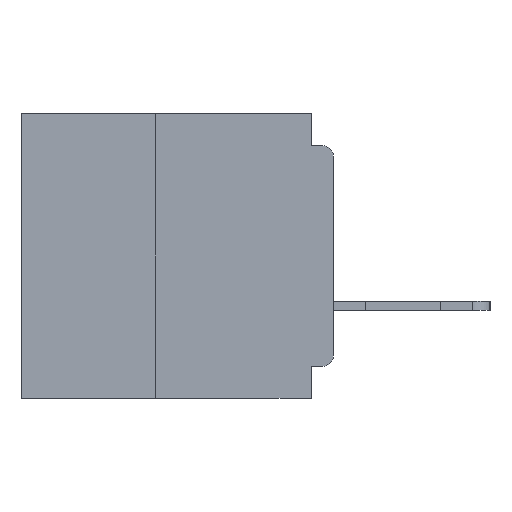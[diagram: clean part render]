
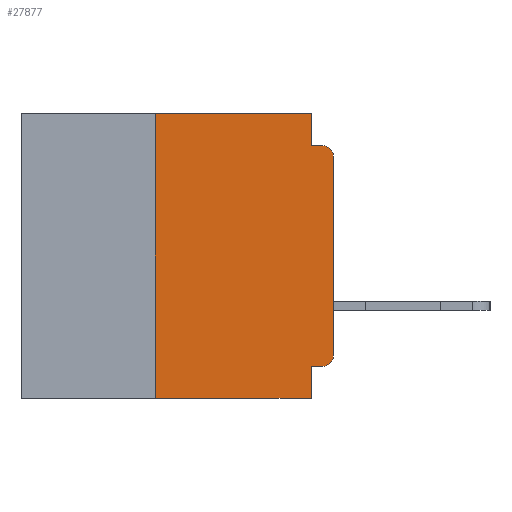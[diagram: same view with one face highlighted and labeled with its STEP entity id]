
A CAD part, left-side view. The second image highlights one B-rep face of the part: STEP entity #27877.
In plain terms, the highlighted planar face has unit normal (-1, 0, 0).
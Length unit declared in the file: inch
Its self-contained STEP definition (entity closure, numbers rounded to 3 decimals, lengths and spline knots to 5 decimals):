
#2453 = DIRECTION ( 'NONE',  ( 0., 0., -1. ) ) ;
#2517 = LINE ( 'NONE', #8392, #47745 ) ;
#2806 = VERTEX_POINT ( 'NONE', #10183 ) ;
#2852 = CARTESIAN_POINT ( 'NONE',  ( 0., 0.25, 0. ) ) ;
#3042 = ORIENTED_EDGE ( 'NONE', *, *, #9630, .F. ) ;
#3552 = DIRECTION ( 'NONE',  ( 0., 0., -1. ) ) ;
#3826 = VERTEX_POINT ( 'NONE', #6297 ) ;
#5851 = LINE ( 'NONE', #14677, #27881 ) ;
#5991 = LINE ( 'NONE', #32245, #39571 ) ;
#6101 = VECTOR ( 'NONE', #44183, 39.37008 ) ;
#6297 = CARTESIAN_POINT ( 'NONE',  ( 0., 0.031, -0.355 ) ) ;
#6954 = VECTOR ( 'NONE', #3552, 39.37008 ) ;
#7157 = DIRECTION ( 'NONE',  ( 1., 0., 0. ) ) ;
#7499 = LINE ( 'NONE', #39809, #6101 ) ;
#8038 = CARTESIAN_POINT ( 'NONE',  ( 0., 0.031, 0. ) ) ;
#8392 = CARTESIAN_POINT ( 'NONE',  ( 0., 0.437, -0.4 ) ) ;
#9630 = EDGE_CURVE ( 'NONE', #53029, #47740, #51088, .T. ) ;
#10183 = CARTESIAN_POINT ( 'NONE',  ( 0., 0., -0.06 ) ) ;
#11050 = LINE ( 'NONE', #43414, #21374 ) ;
#11082 = CARTESIAN_POINT ( 'NONE',  ( 0., 0., -0.34 ) ) ;
#11758 = EDGE_CURVE ( 'NONE', #47740, #37006, #5851, .T. ) ;
#13208 = CARTESIAN_POINT ( 'NONE',  ( 0., 0.015, -0.34 ) ) ;
#14677 = CARTESIAN_POINT ( 'NONE',  ( 0., 0.437, 0. ) ) ;
#16245 = EDGE_LOOP ( 'NONE', ( #28525, #27925, #49879, #46525, #18513, #3042, #54844, #49669, #50476, #22809 ) ) ;
#16630 = VERTEX_POINT ( 'NONE', #11082 ) ;
#17593 = DIRECTION ( 'NONE',  ( 0., 0., -1. ) ) ;
#17692 = VECTOR ( 'NONE', #27886, 39.37008 ) ;
#18513 = ORIENTED_EDGE ( 'NONE', *, *, #11758, .F. ) ;
#20259 = PLANE ( 'NONE',  #42384 ) ;
#21374 = VECTOR ( 'NONE', #26092, 39.37008 ) ;
#21767 = EDGE_CURVE ( 'NONE', #16630, #2806, #7499, .T. ) ;
#22051 = CARTESIAN_POINT ( 'NONE',  ( 0., 0.031, -0.045 ) ) ;
#22265 = CARTESIAN_POINT ( 'NONE',  ( 0., 0.031, 0. ) ) ;
#22636 = VERTEX_POINT ( 'NONE', #22051 ) ;
#22786 = EDGE_CURVE ( 'NONE', #22636, #25768, #42987, .T. ) ;
#22809 = ORIENTED_EDGE ( 'NONE', *, *, #49130, .T. ) ;
#23468 = EDGE_CURVE ( 'NONE', #35784, #3826, #5991, .T. ) ;
#25768 = VERTEX_POINT ( 'NONE', #34960 ) ;
#26092 = DIRECTION ( 'NONE',  ( 0., 0., -1. ) ) ;
#26818 = EDGE_CURVE ( 'NONE', #37006, #22636, #41891, .T. ) ;
#27877 = ADVANCED_FACE ( 'NONE', ( #49863 ), #20259, .F. ) ;
#27881 = VECTOR ( 'NONE', #53741, 39.37008 ) ;
#27886 = DIRECTION ( 'NONE',  ( 0., 0., 1. ) ) ;
#27925 = ORIENTED_EDGE ( 'NONE', *, *, #44469, .T. ) ;
#28525 = ORIENTED_EDGE ( 'NONE', *, *, #21767, .T. ) ;
#28839 = DIRECTION ( 'NONE',  ( -1., 0., 0. ) ) ;
#29574 = VERTEX_POINT ( 'NONE', #37457 ) ;
#32075 = CIRCLE ( 'NONE', #38379, 0.015 ) ;
#32245 = CARTESIAN_POINT ( 'NONE',  ( 0., 0., -0.355 ) ) ;
#33417 = CARTESIAN_POINT ( 'NONE',  ( 0., 0.437, 0. ) ) ;
#34960 = CARTESIAN_POINT ( 'NONE',  ( 0., 0.015, -0.045 ) ) ;
#35622 = CARTESIAN_POINT ( 'NONE',  ( 0., 0.015, -0.355 ) ) ;
#35784 = VERTEX_POINT ( 'NONE', #35622 ) ;
#36368 = AXIS2_PLACEMENT_3D ( 'NONE', #54890, #28839, #2453 ) ;
#37006 = VERTEX_POINT ( 'NONE', #22265 ) ;
#37457 = CARTESIAN_POINT ( 'NONE',  ( 0., 0.031, -0.4 ) ) ;
#37802 = DIRECTION ( 'NONE',  ( 0., 0., -1. ) ) ;
#38379 = AXIS2_PLACEMENT_3D ( 'NONE', #13208, #43721, #17593 ) ;
#39571 = VECTOR ( 'NONE', #49326, 39.37008 ) ;
#39809 = CARTESIAN_POINT ( 'NONE',  ( 0., 0., 0. ) ) ;
#40492 = CARTESIAN_POINT ( 'NONE',  ( 0., 0., -0.045 ) ) ;
#41449 = EDGE_CURVE ( 'NONE', #3826, #29574, #11050, .T. ) ;
#41891 = LINE ( 'NONE', #8038, #6954 ) ;
#42384 = AXIS2_PLACEMENT_3D ( 'NONE', #33417, #7157, #37802 ) ;
#42987 = LINE ( 'NONE', #40492, #45701 ) ;
#43414 = CARTESIAN_POINT ( 'NONE',  ( 0., 0.031, -0.4 ) ) ;
#43481 = EDGE_CURVE ( 'NONE', #53029, #29574, #2517, .T. ) ;
#43721 = DIRECTION ( 'NONE',  ( -1., 0., 0. ) ) ;
#44183 = DIRECTION ( 'NONE',  ( 0., 0., 1. ) ) ;
#44469 = EDGE_CURVE ( 'NONE', #2806, #25768, #51021, .T. ) ;
#45701 = VECTOR ( 'NONE', #49016, 39.37008 ) ;
#46525 = ORIENTED_EDGE ( 'NONE', *, *, #26818, .F. ) ;
#47740 = VERTEX_POINT ( 'NONE', #2852 ) ;
#47745 = VECTOR ( 'NONE', #52310, 39.37008 ) ;
#49016 = DIRECTION ( 'NONE',  ( 0., -1., 0. ) ) ;
#49130 = EDGE_CURVE ( 'NONE', #35784, #16630, #32075, .T. ) ;
#49326 = DIRECTION ( 'NONE',  ( 0., 1., 0. ) ) ;
#49669 = ORIENTED_EDGE ( 'NONE', *, *, #41449, .F. ) ;
#49863 = FACE_OUTER_BOUND ( 'NONE', #16245, .T. ) ;
#49879 = ORIENTED_EDGE ( 'NONE', *, *, #22786, .F. ) ;
#50476 = ORIENTED_EDGE ( 'NONE', *, *, #23468, .F. ) ;
#51021 = CIRCLE ( 'NONE', #36368, 0.015 ) ;
#51088 = LINE ( 'NONE', #53906, #17692 ) ;
#52310 = DIRECTION ( 'NONE',  ( 0., -1., 0. ) ) ;
#53029 = VERTEX_POINT ( 'NONE', #55815 ) ;
#53741 = DIRECTION ( 'NONE',  ( 0., -1., 0. ) ) ;
#53906 = CARTESIAN_POINT ( 'NONE',  ( 0., 0.25, -0.4 ) ) ;
#54844 = ORIENTED_EDGE ( 'NONE', *, *, #43481, .T. ) ;
#54890 = CARTESIAN_POINT ( 'NONE',  ( 0., 0.015, -0.06 ) ) ;
#55815 = CARTESIAN_POINT ( 'NONE',  ( 0., 0.25, -0.4 ) ) ;
